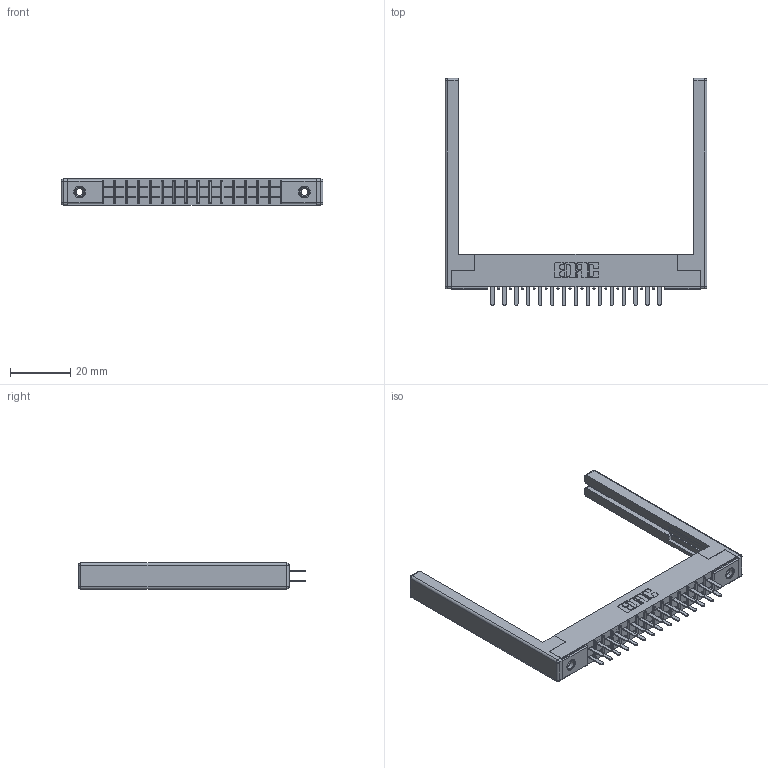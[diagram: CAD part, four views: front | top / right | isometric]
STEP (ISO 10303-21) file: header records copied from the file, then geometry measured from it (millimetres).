
FILE_DESCRIPTION (( 'STEP AP203' ), '1' );
FILE_NAME ('305-030-520-568.STEP', '2019-09-09T16:07:29', ( '' ), ( '' ), 'SwSTEP 2.0', 'SolidWorks 2016', '' );
FILE_SCHEMA (( 'CONFIG_CONTROL_DESIGN' ));
Length unit declared in the file: inch
Products named in the file (5): 305-030-520-568; 307-220-068; 345-250-001_345-250-001-102; 305 Part_.156 Dia; 305-290-001_520
Assembly tree (35 placements, depth 2):
  305-030-520-568
    305 Part_.156 Dia
    305-290-001_520  x30
    345-250-001_345-250-001-102  x2
    307-220-068  x2
Bounding box: 86.87 x 75.39 x 8.71 mm (x, y, z)
Volume: 9816.4 mm3; surface area: 14022.4 mm2
Topology: 35 solids, 35 shells, 1650 faces, 4651 edges, 2998 vertices
Faces by surface type: plane 966, cylinder 600, sphere 68, cone 12, torus 4
Entity records: 22167 total; most frequent: CARTESIAN_POINT 3640, ORIENTED_EDGE 3600, DIRECTION 3562, EDGE_CURVE 1800, LINE 1418, VECTOR 1418, VERTEX_POINT 1150, AXIS2_PLACEMENT_3D 1072
